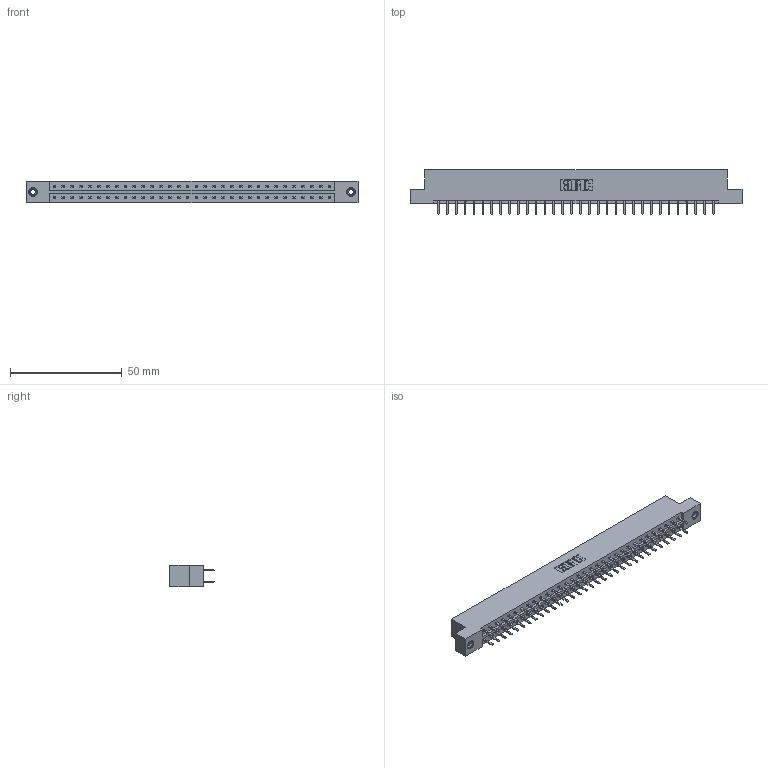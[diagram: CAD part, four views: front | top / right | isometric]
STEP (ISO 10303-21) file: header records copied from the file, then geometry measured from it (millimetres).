
FILE_DESCRIPTION (( 'STEP AP203' ), '1' );
FILE_NAME ('333-064-520-208.STEP', '2018-08-04T09:28:02', ( '' ), ( '' ), 'SwSTEP 2.0', 'SolidWorks 2016', '' );
FILE_SCHEMA (( 'CONFIG_CONTROL_DESIGN' ));
Length unit declared in the file: inch
Products named in the file (4): 333 Part_Flush - .156 Dia - TI; 345-292-001_345-293-120; 345-250-001_345-250-003-102; 333-064-520-208
Assembly tree (67 placements, depth 2):
  333-064-520-208
    333 Part_Flush - .156 Dia - TI
    345-292-001_345-293-120  x64
    345-250-001_345-250-003-102  x2
Bounding box: 148.34 x 20.02 x 9.4 mm (x, y, z)
Volume: 15016.1 mm3; surface area: 17592.5 mm2
Topology: 67 solids, 67 shells, 3758 faces, 10879 edges, 7074 vertices
Faces by surface type: plane 2534, cylinder 1208, cone 12, torus 4
Entity records: 23180 total; most frequent: CARTESIAN_POINT 3849, ORIENTED_EDGE 3766, DIRECTION 3325, EDGE_CURVE 1883, LINE 1731, VECTOR 1731, VERTEX_POINT 1248, AXIS2_PLACEMENT_3D 797
